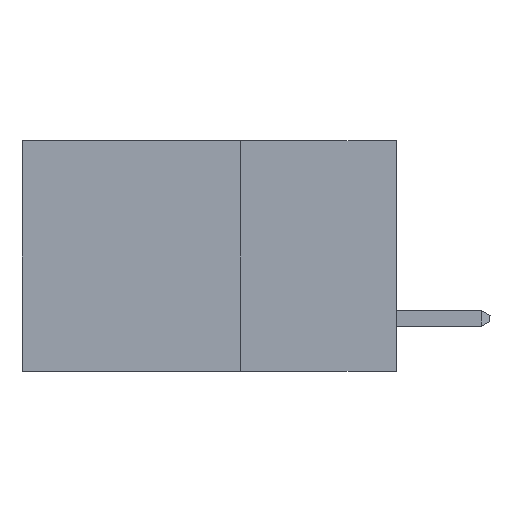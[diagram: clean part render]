
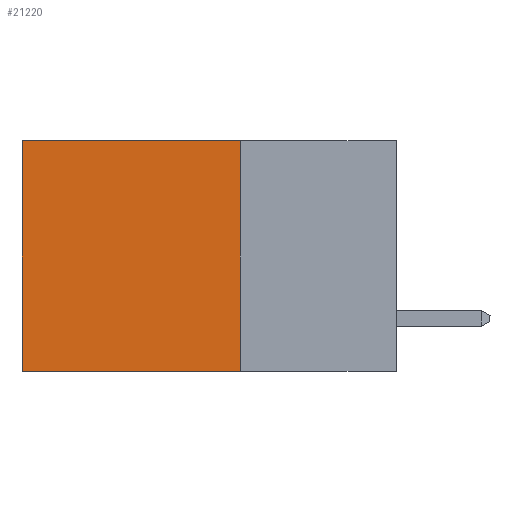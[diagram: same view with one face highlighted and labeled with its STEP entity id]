
A CAD part, left-side view. The second image highlights one B-rep face of the part: STEP entity #21220.
In plain terms, the highlighted planar face has unit normal (-1, 0, 0).
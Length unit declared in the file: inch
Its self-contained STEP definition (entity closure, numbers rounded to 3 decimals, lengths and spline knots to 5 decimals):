
#102 = AXIS2_PLACEMENT_3D ( 'NONE', #6017, #533, #18397 ) ;
#345 = CARTESIAN_POINT ( 'NONE',  ( 0.2615, 0.25, -0.37 ) ) ;
#533 = DIRECTION ( 'NONE',  ( 1., 0., 0. ) ) ;
#848 = VECTOR ( 'NONE', #8795, 39.37008 ) ;
#1878 = LINE ( 'NONE', #345, #10649 ) ;
#2472 = ORIENTED_EDGE ( 'NONE', *, *, #20528, .F. ) ;
#3380 = VECTOR ( 'NONE', #17302, 39.37008 ) ;
#4444 = EDGE_CURVE ( 'NONE', #18228, #20411, #8858, .T. ) ;
#5198 = ORIENTED_EDGE ( 'NONE', *, *, #14624, .T. ) ;
#6017 = CARTESIAN_POINT ( 'NONE',  ( 0.2615, 0.25, -0.37 ) ) ;
#7619 = DIRECTION ( 'NONE',  ( 0., 0., -1. ) ) ;
#8795 = DIRECTION ( 'NONE',  ( 0., 1., 0. ) ) ;
#8858 = LINE ( 'NONE', #16118, #10055 ) ;
#10055 = VECTOR ( 'NONE', #12546, 39.37008 ) ;
#10649 = VECTOR ( 'NONE', #7619, 39.37008 ) ;
#11128 = EDGE_LOOP ( 'NONE', ( #5198, #2472, #14343, #18786 ) ) ;
#11684 = VERTEX_POINT ( 'NONE', #17227 ) ;
#12546 = DIRECTION ( 'NONE',  ( 0., 1., 0. ) ) ;
#12838 = CARTESIAN_POINT ( 'NONE',  ( 0.2615, 0.6, -0.37 ) ) ;
#13645 = EDGE_CURVE ( 'NONE', #18228, #11684, #1878, .T. ) ;
#14343 = ORIENTED_EDGE ( 'NONE', *, *, #13645, .F. ) ;
#14624 = EDGE_CURVE ( 'NONE', #20411, #15258, #20601, .T. ) ;
#15258 = VERTEX_POINT ( 'NONE', #12838 ) ;
#16118 = CARTESIAN_POINT ( 'NONE',  ( 0.2615, 0.25, 0. ) ) ;
#16177 = CARTESIAN_POINT ( 'NONE',  ( 0.2615, 0.25, -0.37 ) ) ;
#16861 = FACE_OUTER_BOUND ( 'NONE', #11128, .T. ) ;
#17227 = CARTESIAN_POINT ( 'NONE',  ( 0.2615, 0.25, -0.37 ) ) ;
#17302 = DIRECTION ( 'NONE',  ( 0., 0., -1. ) ) ;
#17602 = CARTESIAN_POINT ( 'NONE',  ( 0.2615, 0.6, 0. ) ) ;
#18228 = VERTEX_POINT ( 'NONE', #22761 ) ;
#18397 = DIRECTION ( 'NONE',  ( 0., 0., -1. ) ) ;
#18786 = ORIENTED_EDGE ( 'NONE', *, *, #4444, .T. ) ;
#19633 = LINE ( 'NONE', #16177, #848 ) ;
#20411 = VERTEX_POINT ( 'NONE', #17602 ) ;
#20528 = EDGE_CURVE ( 'NONE', #11684, #15258, #19633, .T. ) ;
#20601 = LINE ( 'NONE', #22503, #3380 ) ;
#21220 = ADVANCED_FACE ( 'NONE', ( #16861 ), #22311, .F. ) ;
#22311 = PLANE ( 'NONE',  #102 ) ;
#22503 = CARTESIAN_POINT ( 'NONE',  ( 0.2615, 0.6, -0.37 ) ) ;
#22761 = CARTESIAN_POINT ( 'NONE',  ( 0.2615, 0.25, 0. ) ) ;
